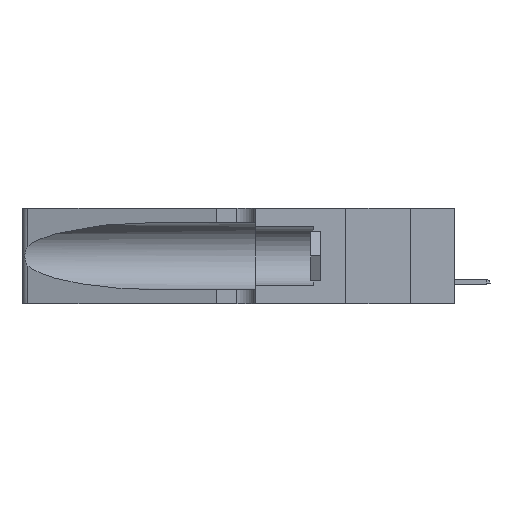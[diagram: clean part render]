
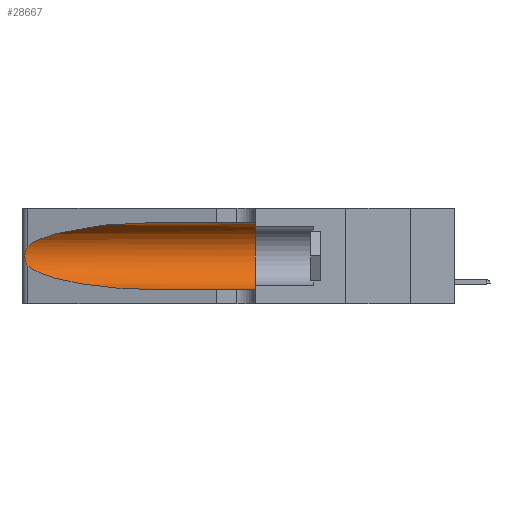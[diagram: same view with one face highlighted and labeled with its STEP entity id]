
A CAD part, left-side view. The second image highlights one B-rep face of the part: STEP entity #28667.
In plain terms, the highlighted cylindrical face has radius 3.308 mm (diameter 6.617 mm), a partial arc.
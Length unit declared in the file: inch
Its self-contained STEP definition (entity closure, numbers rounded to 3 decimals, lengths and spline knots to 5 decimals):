
#894 = CARTESIAN_POINT ( 'NONE',  ( 0.25555, 1.22993, 0.14849 ) ) ;
#1143 = CARTESIAN_POINT ( 'NONE',  ( 0.25787, 1.23484, 0.2124 ) ) ;
#4644 = EDGE_CURVE ( 'NONE', #14110, #42494, #41960, .T. ) ;
#5190 = CARTESIAN_POINT ( 'NONE',  ( 0.25854, 1.2359, 0.20912 ) ) ;
#7295 = CARTESIAN_POINT ( 'NONE',  ( 0.2373, 1.15595, 0.08982 ) ) ;
#7991 = CARTESIAN_POINT ( 'NONE',  ( 0.25789, 1.23486, 0.15765 ) ) ;
#8113 = VERTEX_POINT ( 'NONE', #19431 ) ;
#8494 = CARTESIAN_POINT ( 'NONE',  ( 0.25487, 1.22718, 0.22369 ) ) ;
#8725 = B_SPLINE_CURVE_WITH_KNOTS ( 'NONE', 3,
 ( #8494, #15847, #12038, #1143, #5190, #42680, #28207, #16599, #24176, #46987, #7991, #43680, #894, #9001 ),
 .UNSPECIFIED., .F., .F.,
 ( 4, 2, 2, 2, 2, 2, 4 ),
 ( 0., 0.00027, 0.00053, 0.00107, 0.0016, 0.00187, 0.00214 ),
 .UNSPECIFIED. ) ;
#9001 = CARTESIAN_POINT ( 'NONE',  ( 0.25487, 1.22718, 0.14631 ) ) ;
#9507 = VECTOR ( 'NONE', #30501, 39.37008 ) ;
#10420 = ORIENTED_EDGE ( 'NONE', *, *, #35613, .T. ) ;
#10707 = CARTESIAN_POINT ( 'NONE',  ( 0.25487, 1.22718, 0.22369 ) ) ;
#11503 = CARTESIAN_POINT ( 'NONE',  ( 0.1305, 1.61858, 0.05475 ) ) ;
#11625 = CARTESIAN_POINT ( 'NONE',  ( 0.1305, 0.35, 0.05475 ) ) ;
#12038 = CARTESIAN_POINT ( 'NONE',  ( 0.25639, 1.23184, 0.21858 ) ) ;
#13456 = CIRCLE ( 'NONE', #31263, 0.13025 ) ;
#13684 = DIRECTION ( 'NONE',  ( 0., 0., -1. ) ) ;
#14110 = VERTEX_POINT ( 'NONE', #19776 ) ;
#14828 = LINE ( 'NONE', #11503, #21943 ) ;
#15195 = CARTESIAN_POINT ( 'NONE',  ( 0.25487, 1.22718, 0.14631 ) ) ;
#15218 = ORIENTED_EDGE ( 'NONE', *, *, #41909, .F. ) ;
#15305 = LINE ( 'NONE', #49976, #9507 ) ;
#15847 = CARTESIAN_POINT ( 'NONE',  ( 0.25555, 1.22994, 0.2215 ) ) ;
#16599 = CARTESIAN_POINT ( 'NONE',  ( 0.26075, 1.23896, 0.178 ) ) ;
#18001 = FACE_OUTER_BOUND ( 'NONE', #49174, .T. ) ;
#18285 = CARTESIAN_POINT ( 'NONE',  ( 0.18966, 0.96281, 0.31525 ) ) ;
#18971 = VERTEX_POINT ( 'NONE', #15195 ) ;
#19396 = CARTESIAN_POINT ( 'NONE',  ( 0.25487, 1.22718, 0.22369 ) ) ;
#19431 = CARTESIAN_POINT ( 'NONE',  ( 0.1305, 0.35, 0.31525 ) ) ;
#19776 = CARTESIAN_POINT ( 'NONE',  ( 0.1305, 0.72297, 0.31525 ) ) ;
#20366 = ORIENTED_EDGE ( 'NONE', *, *, #4644, .T. ) ;
#21090 = CARTESIAN_POINT ( 'NONE',  ( 0.1305, 0.72297, 0.05475 ) ) ;
#21943 = VECTOR ( 'NONE', #49502, 39.37008 ) ;
#22280 = VERTEX_POINT ( 'NONE', #11625 ) ;
#22480 = EDGE_CURVE ( 'NONE', #29358, #22280, #14828, .T. ) ;
#22482 = CARTESIAN_POINT ( 'NONE',  ( 0.25487, 1.22718, 0.14631 ) ) ;
#24176 = CARTESIAN_POINT ( 'NONE',  ( 0.26017, 1.23833, 0.17102 ) ) ;
#25078 = CYLINDRICAL_SURFACE ( 'NONE', #46760, 0.13025 ) ;
#25966 = CARTESIAN_POINT ( 'NONE',  ( 0.1305, 0.35, 0.185 ) ) ;
#27875 = EDGE_CURVE ( 'NONE', #14110, #8113, #15305, .T. ) ;
#28207 = CARTESIAN_POINT ( 'NONE',  ( 0.26075, 1.23896, 0.19203 ) ) ;
#28667 = ADVANCED_FACE ( 'NONE', ( #18001 ), #25078, .F. ) ;
#29358 = VERTEX_POINT ( 'NONE', #21090 ) ;
#30501 = DIRECTION ( 'NONE',  ( 0., -1., 0. ) ) ;
#31263 = AXIS2_PLACEMENT_3D ( 'NONE', #25966, #49249, #42162 ) ;
#32822 = ORIENTED_EDGE ( 'NONE', *, *, #27875, .F. ) ;
#33240 =( BOUNDED_CURVE ( )  B_SPLINE_CURVE ( 3, ( #22482, #7295, #33892, #49350 ),
 .UNSPECIFIED., .F., .F. ) 
 B_SPLINE_CURVE_WITH_KNOTS ( ( 4, 4 ),
 ( 3.44316, 4.71239 ),
 .UNSPECIFIED. ) 
 CURVE ( )  GEOMETRIC_REPRESENTATION_ITEM ( )  RATIONAL_B_SPLINE_CURVE ( ( 1., 0.87, 0.87, 1. ) ) 
 REPRESENTATION_ITEM ( '' )  );
#33892 = CARTESIAN_POINT ( 'NONE',  ( 0.18966, 0.96281, 0.05475 ) ) ;
#35613 = EDGE_CURVE ( 'NONE', #18971, #29358, #33240, .T. ) ;
#41657 = EDGE_CURVE ( 'NONE', #42494, #18971, #8725, .T. ) ;
#41909 = EDGE_CURVE ( 'NONE', #8113, #22280, #13456, .T. ) ;
#41960 =( BOUNDED_CURVE ( )  B_SPLINE_CURVE ( 3, ( #45400, #18285, #49180, #10707 ),
 .UNSPECIFIED., .F., .F. ) 
 B_SPLINE_CURVE_WITH_KNOTS ( ( 4, 4 ),
 ( 1.5708, 2.84003 ),
 .UNSPECIFIED. ) 
 CURVE ( )  GEOMETRIC_REPRESENTATION_ITEM ( )  RATIONAL_B_SPLINE_CURVE ( ( 1., 0.87, 0.87, 1. ) ) 
 REPRESENTATION_ITEM ( '' )  );
#42162 = DIRECTION ( 'NONE',  ( 0., 0., 1. ) ) ;
#42494 = VERTEX_POINT ( 'NONE', #19396 ) ;
#42680 = CARTESIAN_POINT ( 'NONE',  ( 0.26018, 1.23835, 0.19895 ) ) ;
#43680 = CARTESIAN_POINT ( 'NONE',  ( 0.25639, 1.23186, 0.15144 ) ) ;
#44013 = ORIENTED_EDGE ( 'NONE', *, *, #41657, .T. ) ;
#45400 = CARTESIAN_POINT ( 'NONE',  ( 0.1305, 0.72297, 0.31525 ) ) ;
#46083 = ORIENTED_EDGE ( 'NONE', *, *, #22480, .T. ) ;
#46760 = AXIS2_PLACEMENT_3D ( 'NONE', #48121, #49804, #13684 ) ;
#46987 = CARTESIAN_POINT ( 'NONE',  ( 0.25856, 1.23593, 0.16098 ) ) ;
#48121 = CARTESIAN_POINT ( 'NONE',  ( 0.1305, 1.61858, 0.185 ) ) ;
#49174 = EDGE_LOOP ( 'NONE', ( #20366, #44013, #10420, #46083, #15218, #32822 ) ) ;
#49180 = CARTESIAN_POINT ( 'NONE',  ( 0.2373, 1.15595, 0.28018 ) ) ;
#49249 = DIRECTION ( 'NONE',  ( 0., 1., 0. ) ) ;
#49350 = CARTESIAN_POINT ( 'NONE',  ( 0.1305, 0.72297, 0.05475 ) ) ;
#49502 = DIRECTION ( 'NONE',  ( 0., -1., 0. ) ) ;
#49804 = DIRECTION ( 'NONE',  ( 0., -1., 0. ) ) ;
#49976 = CARTESIAN_POINT ( 'NONE',  ( 0.1305, 1.61858, 0.31525 ) ) ;
